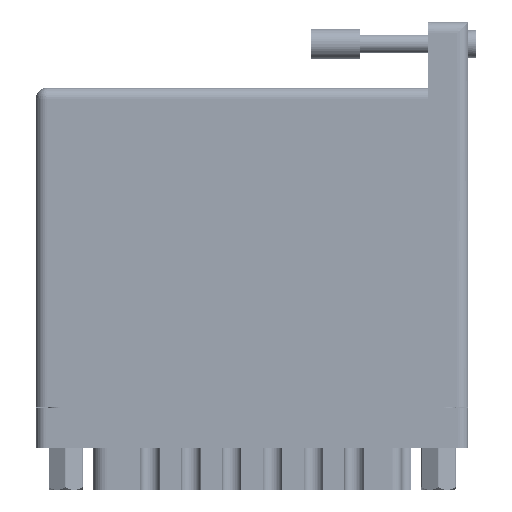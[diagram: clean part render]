
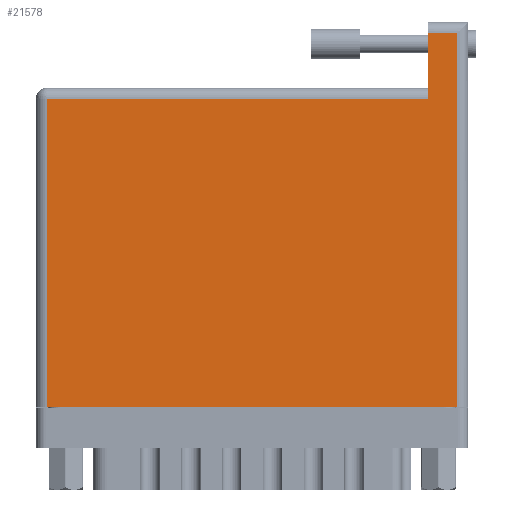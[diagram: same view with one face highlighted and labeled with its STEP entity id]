
A CAD part, front view. The second image highlights one B-rep face of the part: STEP entity #21578.
In plain terms, the highlighted face is planar.
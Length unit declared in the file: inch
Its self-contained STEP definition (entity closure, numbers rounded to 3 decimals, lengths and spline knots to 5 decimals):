
#573 = VECTOR ( 'NONE', #46511, 39.37008 ) ;
#3138 = LINE ( 'NONE', #14964, #573 ) ;
#4284 = VECTOR ( 'NONE', #7259, 39.37008 ) ;
#4936 = EDGE_CURVE ( 'NONE', #89511, #77486, #38840, .T. ) ;
#7259 = DIRECTION ( 'NONE',  ( 0., -1., 0. ) ) ;
#7828 = CARTESIAN_POINT ( 'NONE',  ( 0., 2.03, 0. ) ) ;
#8564 = CARTESIAN_POINT ( 'NONE',  ( 2.685, 2.38, 0. ) ) ;
#14964 = CARTESIAN_POINT ( 'NONE',  ( 2.685, 2.45, 0. ) ) ;
#17118 = VECTOR ( 'NONE', #85812, 39.37008 ) ;
#20760 = LINE ( 'NONE', #28162, #89942 ) ;
#21578 = ADVANCED_FACE ( 'NONE', ( #81707 ), #72324, .F. ) ;
#21978 = AXIS2_PLACEMENT_3D ( 'NONE', #7828, #88689, #73371 ) ;
#23239 = VERTEX_POINT ( 'NONE', #49822 ) ;
#28162 = CARTESIAN_POINT ( 'NONE',  ( 2.499, 2.45, 0. ) ) ;
#30136 = DIRECTION ( 'NONE',  ( -1., 0., 0. ) ) ;
#38840 = LINE ( 'NONE', #85461, #17118 ) ;
#41406 = ORIENTED_EDGE ( 'NONE', *, *, #97615, .T. ) ;
#43696 = VERTEX_POINT ( 'NONE', #77039 ) ;
#44889 = ORIENTED_EDGE ( 'NONE', *, *, #4936, .T. ) ;
#46511 = DIRECTION ( 'NONE',  ( 0., 1., 0. ) ) ;
#46764 = VECTOR ( 'NONE', #92669, 39.37008 ) ;
#49822 = CARTESIAN_POINT ( 'NONE',  ( 0.07, 0., 0. ) ) ;
#50363 = LINE ( 'NONE', #56322, #4284 ) ;
#50655 = EDGE_CURVE ( 'NONE', #77486, #103697, #20760, .T. ) ;
#55434 = CARTESIAN_POINT ( 'NONE',  ( 2.499, 2.38, 0. ) ) ;
#56322 = CARTESIAN_POINT ( 'NONE',  ( 0.07, 0., 0. ) ) ;
#56455 = VECTOR ( 'NONE', #30136, 39.37008 ) ;
#69892 = ORIENTED_EDGE ( 'NONE', *, *, #50655, .T. ) ;
#72324 = PLANE ( 'NONE',  #21978 ) ;
#73371 = DIRECTION ( 'NONE',  ( -1., 0., 0. ) ) ;
#75114 = ORIENTED_EDGE ( 'NONE', *, *, #85366, .T. ) ;
#76943 = CARTESIAN_POINT ( 'NONE',  ( 0., 0., 0. ) ) ;
#77039 = CARTESIAN_POINT ( 'NONE',  ( 0.07, 1.96, 0. ) ) ;
#77064 = CARTESIAN_POINT ( 'NONE',  ( 2.685, 0., 0. ) ) ;
#77486 = VERTEX_POINT ( 'NONE', #55434 ) ;
#78875 = LINE ( 'NONE', #76943, #46764 ) ;
#80763 = LINE ( 'NONE', #96426, #56455 ) ;
#81108 = ORIENTED_EDGE ( 'NONE', *, *, #102012, .T. ) ;
#81707 = FACE_OUTER_BOUND ( 'NONE', #86391, .T. ) ;
#85366 = EDGE_CURVE ( 'NONE', #23239, #87791, #78875, .T. ) ;
#85461 = CARTESIAN_POINT ( 'NONE',  ( 0., 2.38, 0. ) ) ;
#85812 = DIRECTION ( 'NONE',  ( -1., 0., 0. ) ) ;
#86391 = EDGE_LOOP ( 'NONE', ( #69892, #41406, #81108, #75114, #105613, #44889 ) ) ;
#87791 = VERTEX_POINT ( 'NONE', #77064 ) ;
#88689 = DIRECTION ( 'NONE',  ( 0., 0., -1. ) ) ;
#89511 = VERTEX_POINT ( 'NONE', #8564 ) ;
#89942 = VECTOR ( 'NONE', #92344, 39.37008 ) ;
#92344 = DIRECTION ( 'NONE',  ( 0., -1., 0. ) ) ;
#92669 = DIRECTION ( 'NONE',  ( 1., 0., 0. ) ) ;
#95998 = CARTESIAN_POINT ( 'NONE',  ( 2.499, 1.96, 0. ) ) ;
#96426 = CARTESIAN_POINT ( 'NONE',  ( 0., 1.96, 0. ) ) ;
#97615 = EDGE_CURVE ( 'NONE', #103697, #43696, #80763, .T. ) ;
#102012 = EDGE_CURVE ( 'NONE', #43696, #23239, #50363, .T. ) ;
#103697 = VERTEX_POINT ( 'NONE', #95998 ) ;
#104992 = EDGE_CURVE ( 'NONE', #87791, #89511, #3138, .T. ) ;
#105613 = ORIENTED_EDGE ( 'NONE', *, *, #104992, .T. ) ;
